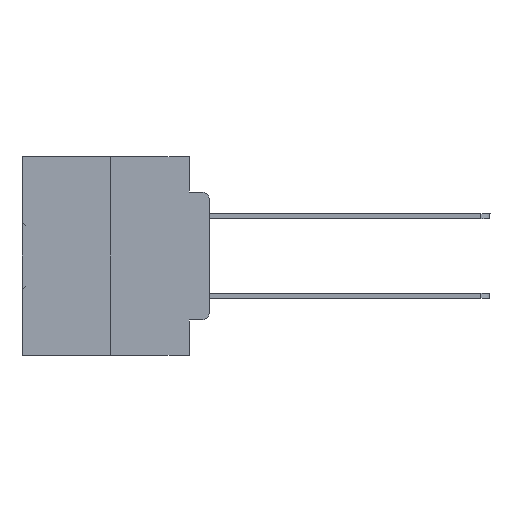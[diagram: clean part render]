
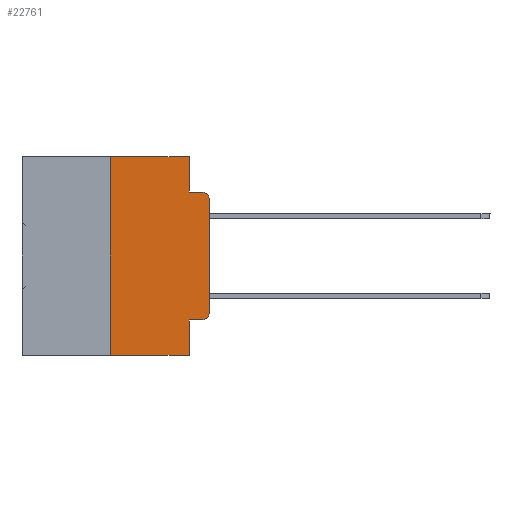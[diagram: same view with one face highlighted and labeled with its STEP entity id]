
A CAD part, left-side view. The second image highlights one B-rep face of the part: STEP entity #22761.
In plain terms, the highlighted planar face has unit normal (-1, 0, 0).
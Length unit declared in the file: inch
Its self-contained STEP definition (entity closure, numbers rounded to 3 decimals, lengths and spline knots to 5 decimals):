
#572 = ORIENTED_EDGE ( 'NONE', *, *, #20939, .T. ) ;
#1738 = VECTOR ( 'NONE', #3015, 39.37008 ) ;
#2430 = VERTEX_POINT ( 'NONE', #4892 ) ;
#3015 = DIRECTION ( 'NONE',  ( 0., 0., 1. ) ) ;
#3168 = DIRECTION ( 'NONE',  ( 0., -1., 0. ) ) ;
#3305 = CARTESIAN_POINT ( 'NONE',  ( 0., 0.051, 0. ) ) ;
#4159 = VECTOR ( 'NONE', #30211, 39.37008 ) ;
#4221 = CARTESIAN_POINT ( 'NONE',  ( 0., 0.051, -0.5 ) ) ;
#4474 = ORIENTED_EDGE ( 'NONE', *, *, #30719, .T. ) ;
#4718 = ORIENTED_EDGE ( 'NONE', *, *, #27050, .T. ) ;
#4892 = CARTESIAN_POINT ( 'NONE',  ( 0., 0.02, -0.0885 ) ) ;
#5009 = ORIENTED_EDGE ( 'NONE', *, *, #27436, .F. ) ;
#5036 = DIRECTION ( 'NONE',  ( 0., 0., -1. ) ) ;
#5400 = CARTESIAN_POINT ( 'NONE',  ( 0., 0.051, -0.0885 ) ) ;
#5624 = CARTESIAN_POINT ( 'NONE',  ( 0., 0.473, -0.5 ) ) ;
#6260 = LINE ( 'NONE', #35449, #33788 ) ;
#6322 = DIRECTION ( 'NONE',  ( 0., 0., -1. ) ) ;
#6731 = AXIS2_PLACEMENT_3D ( 'NONE', #7134, #12749, #30362 ) ;
#6957 = FACE_OUTER_BOUND ( 'NONE', #16564, .T. ) ;
#7134 = CARTESIAN_POINT ( 'NONE',  ( 0., 0.473, 0. ) ) ;
#7412 = CIRCLE ( 'NONE', #20570, 0.02 ) ;
#7658 = LINE ( 'NONE', #33128, #12122 ) ;
#7707 = EDGE_CURVE ( 'NONE', #33654, #2430, #23369, .T. ) ;
#7922 = VERTEX_POINT ( 'NONE', #26750 ) ;
#8326 = EDGE_CURVE ( 'NONE', #32683, #2430, #7412, .T. ) ;
#8428 = LINE ( 'NONE', #5624, #29693 ) ;
#9760 = CARTESIAN_POINT ( 'NONE',  ( 0., 0.473, 0. ) ) ;
#9947 = PLANE ( 'NONE',  #6731 ) ;
#11204 = LINE ( 'NONE', #36673, #23127 ) ;
#11369 = DIRECTION ( 'NONE',  ( -1., 0., 0. ) ) ;
#12122 = VECTOR ( 'NONE', #5036, 39.37008 ) ;
#12394 = EDGE_CURVE ( 'NONE', #36417, #14341, #12756, .T. ) ;
#12690 = DIRECTION ( 'NONE',  ( 0., 0., -1. ) ) ;
#12749 = DIRECTION ( 'NONE',  ( 1., 0., 0. ) ) ;
#12756 = LINE ( 'NONE', #9760, #15195 ) ;
#12886 = CARTESIAN_POINT ( 'NONE',  ( 0., 0.02, -0.1085 ) ) ;
#13462 = DIRECTION ( 'NONE',  ( 0., 0., 1. ) ) ;
#13464 = VERTEX_POINT ( 'NONE', #4221 ) ;
#14341 = VERTEX_POINT ( 'NONE', #3305 ) ;
#14548 = CARTESIAN_POINT ( 'NONE',  ( 0., 0.02, -0.3915 ) ) ;
#15195 = VECTOR ( 'NONE', #36165, 39.37008 ) ;
#15351 = CARTESIAN_POINT ( 'NONE',  ( 0., 0.25, -0.5 ) ) ;
#16564 = EDGE_LOOP ( 'NONE', ( #4474, #33509, #20912, #17292, #30471, #5009, #4718, #32546, #572, #35883 ) ) ;
#16687 = VERTEX_POINT ( 'NONE', #19387 ) ;
#17292 = ORIENTED_EDGE ( 'NONE', *, *, #25063, .F. ) ;
#18402 = CARTESIAN_POINT ( 'NONE',  ( 0., 0.051, -0.4115 ) ) ;
#19387 = CARTESIAN_POINT ( 'NONE',  ( 0., 0.02, -0.4115 ) ) ;
#20570 = AXIS2_PLACEMENT_3D ( 'NONE', #12886, #30304, #12690 ) ;
#20912 = ORIENTED_EDGE ( 'NONE', *, *, #7707, .F. ) ;
#20939 = EDGE_CURVE ( 'NONE', #7922, #16687, #29649, .T. ) ;
#21104 = CARTESIAN_POINT ( 'NONE',  ( 0., 0., -0.1085 ) ) ;
#22761 = ADVANCED_FACE ( 'NONE', ( #6957 ), #9947, .F. ) ;
#22896 = VECTOR ( 'NONE', #3168, 39.37008 ) ;
#23127 = VECTOR ( 'NONE', #13462, 39.37008 ) ;
#23284 = EDGE_CURVE ( 'NONE', #7922, #13464, #7658, .T. ) ;
#23369 = LINE ( 'NONE', #25640, #22896 ) ;
#23431 = EDGE_CURVE ( 'NONE', #16687, #33141, #33683, .T. ) ;
#23458 = DIRECTION ( 'NONE',  ( 0., 0., -1. ) ) ;
#24011 = CARTESIAN_POINT ( 'NONE',  ( 0., 0., -0.3915 ) ) ;
#25063 = EDGE_CURVE ( 'NONE', #14341, #33654, #6260, .T. ) ;
#25640 = CARTESIAN_POINT ( 'NONE',  ( 0., 0.051, -0.0885 ) ) ;
#26750 = CARTESIAN_POINT ( 'NONE',  ( 0., 0.051, -0.4115 ) ) ;
#27050 = EDGE_CURVE ( 'NONE', #36755, #13464, #8428, .T. ) ;
#27436 = EDGE_CURVE ( 'NONE', #36755, #36417, #11204, .T. ) ;
#28304 = LINE ( 'NONE', #31297, #1738 ) ;
#29460 = AXIS2_PLACEMENT_3D ( 'NONE', #14548, #11369, #6322 ) ;
#29649 = LINE ( 'NONE', #18402, #4159 ) ;
#29693 = VECTOR ( 'NONE', #36715, 39.37008 ) ;
#30211 = DIRECTION ( 'NONE',  ( 0., -1., 0. ) ) ;
#30304 = DIRECTION ( 'NONE',  ( -1., 0., 0. ) ) ;
#30362 = DIRECTION ( 'NONE',  ( 0., 0., -1. ) ) ;
#30471 = ORIENTED_EDGE ( 'NONE', *, *, #12394, .F. ) ;
#30719 = EDGE_CURVE ( 'NONE', #33141, #32683, #28304, .T. ) ;
#30937 = CARTESIAN_POINT ( 'NONE',  ( 0., 0.25, 0. ) ) ;
#31297 = CARTESIAN_POINT ( 'NONE',  ( 0., 0., 0. ) ) ;
#32546 = ORIENTED_EDGE ( 'NONE', *, *, #23284, .F. ) ;
#32683 = VERTEX_POINT ( 'NONE', #21104 ) ;
#33128 = CARTESIAN_POINT ( 'NONE',  ( 0., 0.051, 0. ) ) ;
#33141 = VERTEX_POINT ( 'NONE', #24011 ) ;
#33509 = ORIENTED_EDGE ( 'NONE', *, *, #8326, .T. ) ;
#33654 = VERTEX_POINT ( 'NONE', #5400 ) ;
#33683 = CIRCLE ( 'NONE', #29460, 0.02 ) ;
#33788 = VECTOR ( 'NONE', #23458, 39.37008 ) ;
#35449 = CARTESIAN_POINT ( 'NONE',  ( 0., 0.051, 0. ) ) ;
#35883 = ORIENTED_EDGE ( 'NONE', *, *, #23431, .T. ) ;
#36165 = DIRECTION ( 'NONE',  ( 0., -1., 0. ) ) ;
#36417 = VERTEX_POINT ( 'NONE', #30937 ) ;
#36673 = CARTESIAN_POINT ( 'NONE',  ( 0., 0.25, 0. ) ) ;
#36715 = DIRECTION ( 'NONE',  ( 0., -1., 0. ) ) ;
#36755 = VERTEX_POINT ( 'NONE', #15351 ) ;
